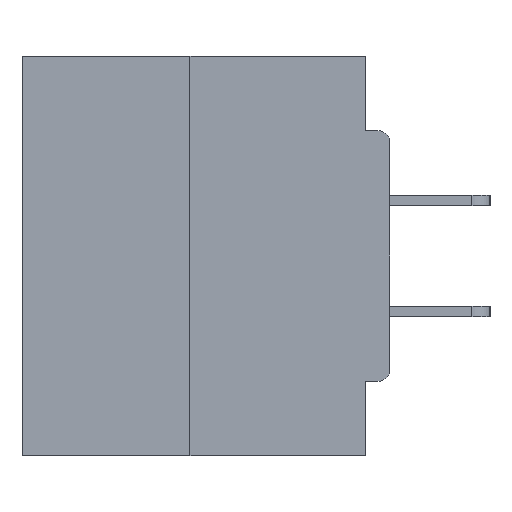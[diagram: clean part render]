
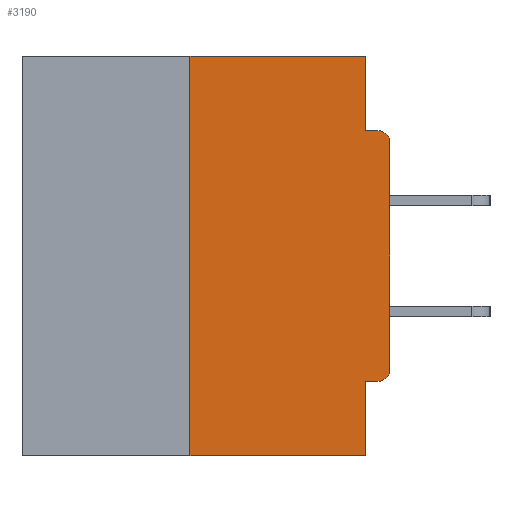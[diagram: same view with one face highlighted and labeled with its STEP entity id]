
A CAD part, left-side view. The second image highlights one B-rep face of the part: STEP entity #3190.
In plain terms, the highlighted planar face has unit normal (-1, 0, 0).
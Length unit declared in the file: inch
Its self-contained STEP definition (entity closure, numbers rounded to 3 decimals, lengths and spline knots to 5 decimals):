
#462 = VERTEX_POINT ( 'NONE', #7999 ) ;
#1194 = CIRCLE ( 'NONE', #21045, 0.015 ) ;
#1292 = FACE_OUTER_BOUND ( 'NONE', #3073, .T. ) ;
#1821 = ORIENTED_EDGE ( 'NONE', *, *, #7043, .F. ) ;
#2415 = EDGE_CURVE ( 'NONE', #27367, #4475, #14155, .T. ) ;
#2538 = CARTESIAN_POINT ( 'NONE',  ( 0., 0.031, -0.5 ) ) ;
#2816 = VERTEX_POINT ( 'NONE', #31583 ) ;
#3073 = EDGE_LOOP ( 'NONE', ( #35575, #34094, #22902, #1821, #20924, #15391, #27316, #35612, #14436, #3893 ) ) ;
#3190 = ADVANCED_FACE ( 'NONE', ( #1292 ), #21227, .F. ) ;
#3455 = VECTOR ( 'NONE', #18899, 39.37008 ) ;
#3893 = ORIENTED_EDGE ( 'NONE', *, *, #4052, .F. ) ;
#4052 = EDGE_CURVE ( 'NONE', #8533, #11385, #9975, .T. ) ;
#4224 = VERTEX_POINT ( 'NONE', #27340 ) ;
#4475 = VERTEX_POINT ( 'NONE', #7016 ) ;
#6077 = EDGE_CURVE ( 'NONE', #2816, #24697, #15309, .T. ) ;
#6081 = VERTEX_POINT ( 'NONE', #23905 ) ;
#7016 = CARTESIAN_POINT ( 'NONE',  ( 0., 0., -0.1085 ) ) ;
#7043 = EDGE_CURVE ( 'NONE', #4224, #25702, #26933, .T. ) ;
#7198 = DIRECTION ( 'NONE',  ( 0., 0., -1. ) ) ;
#7483 = CARTESIAN_POINT ( 'NONE',  ( 0., 0.015, -0.1085 ) ) ;
#7999 = CARTESIAN_POINT ( 'NONE',  ( 0., 0.015, -0.4065 ) ) ;
#8279 = CARTESIAN_POINT ( 'NONE',  ( 0., 0., -0.3915 ) ) ;
#8533 = VERTEX_POINT ( 'NONE', #18051 ) ;
#8647 = CARTESIAN_POINT ( 'NONE',  ( 0., 0., -0.0935 ) ) ;
#9613 = CIRCLE ( 'NONE', #10199, 0.015 ) ;
#9745 = DIRECTION ( 'NONE',  ( 0., -1., 0. ) ) ;
#9917 = CARTESIAN_POINT ( 'NONE',  ( 0., 0.46, -0.5 ) ) ;
#9975 = LINE ( 'NONE', #24067, #15956 ) ;
#10199 = AXIS2_PLACEMENT_3D ( 'NONE', #7483, #35674, #15524 ) ;
#10542 = EDGE_CURVE ( 'NONE', #462, #27367, #1194, .T. ) ;
#11385 = VERTEX_POINT ( 'NONE', #21678 ) ;
#11804 = EDGE_CURVE ( 'NONE', #2816, #25702, #29877, .T. ) ;
#13810 = CARTESIAN_POINT ( 'NONE',  ( 0., 0., -0.4065 ) ) ;
#13976 = CARTESIAN_POINT ( 'NONE',  ( 0., 0., 0. ) ) ;
#14084 = VECTOR ( 'NONE', #33388, 39.37008 ) ;
#14155 = LINE ( 'NONE', #13976, #14084 ) ;
#14267 = DIRECTION ( 'NONE',  ( -1., 0., 0. ) ) ;
#14436 = ORIENTED_EDGE ( 'NONE', *, *, #31607, .F. ) ;
#15130 = CARTESIAN_POINT ( 'NONE',  ( 0., 0.015, -0.3915 ) ) ;
#15211 = VECTOR ( 'NONE', #26284, 39.37008 ) ;
#15309 = LINE ( 'NONE', #17897, #15211 ) ;
#15391 = ORIENTED_EDGE ( 'NONE', *, *, #10542, .T. ) ;
#15524 = DIRECTION ( 'NONE',  ( 0., 0., -1. ) ) ;
#15920 = DIRECTION ( 'NONE',  ( 0., 0., -1. ) ) ;
#15956 = VECTOR ( 'NONE', #18231, 39.37008 ) ;
#17897 = CARTESIAN_POINT ( 'NONE',  ( 0., 0.25, 0. ) ) ;
#18051 = CARTESIAN_POINT ( 'NONE',  ( 0., 0.031, 0. ) ) ;
#18231 = DIRECTION ( 'NONE',  ( 0., 0., -1. ) ) ;
#18899 = DIRECTION ( 'NONE',  ( 0., -1., 0. ) ) ;
#19009 = EDGE_CURVE ( 'NONE', #462, #4224, #27704, .T. ) ;
#20343 = DIRECTION ( 'NONE',  ( 0., -1., 0. ) ) ;
#20924 = ORIENTED_EDGE ( 'NONE', *, *, #19009, .F. ) ;
#21045 = AXIS2_PLACEMENT_3D ( 'NONE', #15130, #14267, #26282 ) ;
#21227 = PLANE ( 'NONE',  #31773 ) ;
#21678 = CARTESIAN_POINT ( 'NONE',  ( 0., 0.031, -0.0935 ) ) ;
#22902 = ORIENTED_EDGE ( 'NONE', *, *, #11804, .T. ) ;
#23905 = CARTESIAN_POINT ( 'NONE',  ( 0., 0.015, -0.0935 ) ) ;
#24067 = CARTESIAN_POINT ( 'NONE',  ( 0., 0.031, 0. ) ) ;
#24697 = VERTEX_POINT ( 'NONE', #27006 ) ;
#24963 = DIRECTION ( 'NONE',  ( 0., 1., 0. ) ) ;
#25702 = VERTEX_POINT ( 'NONE', #2538 ) ;
#26282 = DIRECTION ( 'NONE',  ( 0., 0., -1. ) ) ;
#26284 = DIRECTION ( 'NONE',  ( 0., 0., 1. ) ) ;
#26933 = LINE ( 'NONE', #35401, #29191 ) ;
#27006 = CARTESIAN_POINT ( 'NONE',  ( 0., 0.25, 0. ) ) ;
#27316 = ORIENTED_EDGE ( 'NONE', *, *, #2415, .T. ) ;
#27340 = CARTESIAN_POINT ( 'NONE',  ( 0., 0.031, -0.4065 ) ) ;
#27367 = VERTEX_POINT ( 'NONE', #8279 ) ;
#27704 = LINE ( 'NONE', #13810, #32492 ) ;
#29191 = VECTOR ( 'NONE', #7198, 39.37008 ) ;
#29326 = CARTESIAN_POINT ( 'NONE',  ( 0., 0.46, 0. ) ) ;
#29877 = LINE ( 'NONE', #9917, #3455 ) ;
#29916 = EDGE_CURVE ( 'NONE', #4475, #6081, #9613, .T. ) ;
#31583 = CARTESIAN_POINT ( 'NONE',  ( 0., 0.25, -0.5 ) ) ;
#31607 = EDGE_CURVE ( 'NONE', #11385, #6081, #31707, .T. ) ;
#31707 = LINE ( 'NONE', #8647, #33086 ) ;
#31773 = AXIS2_PLACEMENT_3D ( 'NONE', #32038, #32403, #15920 ) ;
#32038 = CARTESIAN_POINT ( 'NONE',  ( 0., 0.46, 0. ) ) ;
#32403 = DIRECTION ( 'NONE',  ( 1., 0., 0. ) ) ;
#32492 = VECTOR ( 'NONE', #24963, 39.37008 ) ;
#33086 = VECTOR ( 'NONE', #20343, 39.37008 ) ;
#33388 = DIRECTION ( 'NONE',  ( 0., 0., 1. ) ) ;
#34094 = ORIENTED_EDGE ( 'NONE', *, *, #6077, .F. ) ;
#34393 = VECTOR ( 'NONE', #9745, 39.37008 ) ;
#35256 = EDGE_CURVE ( 'NONE', #24697, #8533, #35398, .T. ) ;
#35398 = LINE ( 'NONE', #29326, #34393 ) ;
#35401 = CARTESIAN_POINT ( 'NONE',  ( 0., 0.031, -0.5 ) ) ;
#35575 = ORIENTED_EDGE ( 'NONE', *, *, #35256, .F. ) ;
#35612 = ORIENTED_EDGE ( 'NONE', *, *, #29916, .T. ) ;
#35674 = DIRECTION ( 'NONE',  ( -1., 0., 0. ) ) ;
